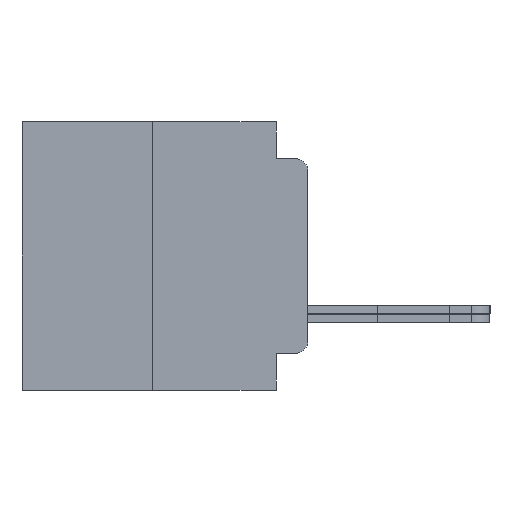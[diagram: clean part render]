
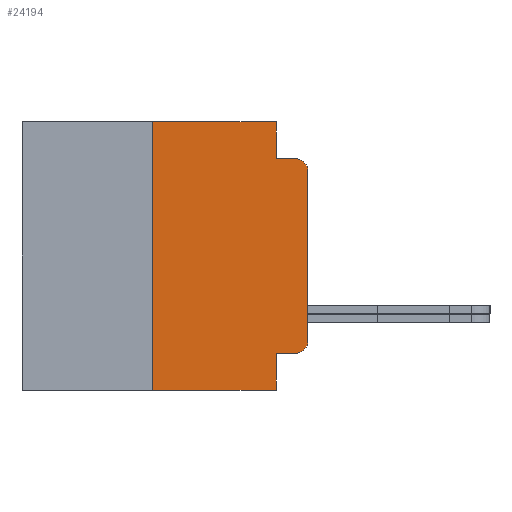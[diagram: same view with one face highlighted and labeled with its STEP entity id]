
A CAD part, left-side view. The second image highlights one B-rep face of the part: STEP entity #24194.
In plain terms, the highlighted planar face has unit normal (-1, 0, 0).
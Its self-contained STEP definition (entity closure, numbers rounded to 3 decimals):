
#92 = CARTESIAN_POINT ( 'NONE',  ( -75.603, 1.295, 0. ) ) ;
#832 = CARTESIAN_POINT ( 'NONE',  ( -75.603, 0., 3.467 ) ) ;
#1432 = DIRECTION ( 'NONE',  ( 1., 0., 0. ) ) ;
#1450 = ORIENTED_EDGE ( 'NONE', *, *, #24512, .F. ) ;
#1784 = VERTEX_POINT ( 'NONE', #21389 ) ;
#1947 = CARTESIAN_POINT ( 'NONE',  ( -75.603, 1.295, -3.975 ) ) ;
#1949 = DIRECTION ( 'NONE',  ( 0., -1., 0. ) ) ;
#2261 = DIRECTION ( 'NONE',  ( 0., 0., -1. ) ) ;
#2635 = VECTOR ( 'NONE', #3875, 1000. ) ;
#3875 = DIRECTION ( 'NONE',  ( 0., 0., -1. ) ) ;
#4479 = CARTESIAN_POINT ( 'NONE',  ( -75.603, 1.295, -3.975 ) ) ;
#4803 = ORIENTED_EDGE ( 'NONE', *, *, #28162, .T. ) ;
#4828 = CARTESIAN_POINT ( 'NONE',  ( -75.603, 6.35, 5.486 ) ) ;
#5490 = DIRECTION ( 'NONE',  ( 0., 0., -1. ) ) ;
#5609 = LINE ( 'NONE', #21966, #27846 ) ;
#6178 = CIRCLE ( 'NONE', #6766, 0.508 ) ;
#6766 = AXIS2_PLACEMENT_3D ( 'NONE', #21391, #14702, #5490 ) ;
#6813 = VERTEX_POINT ( 'NONE', #12914 ) ;
#6880 = VERTEX_POINT ( 'NONE', #13397 ) ;
#7063 = DIRECTION ( 'NONE',  ( 0., -1., 0. ) ) ;
#7454 = ORIENTED_EDGE ( 'NONE', *, *, #24112, .T. ) ;
#7883 = EDGE_CURVE ( 'NONE', #17727, #1784, #21104, .T. ) ;
#8304 = VECTOR ( 'NONE', #10599, 1000. ) ;
#9249 = LINE ( 'NONE', #92, #2635 ) ;
#9313 = VERTEX_POINT ( 'NONE', #4828 ) ;
#9886 = CARTESIAN_POINT ( 'NONE',  ( -75.603, 11.684, -5.486 ) ) ;
#9949 = DIRECTION ( 'NONE',  ( 0., 0., 1. ) ) ;
#10599 = DIRECTION ( 'NONE',  ( 0., 0., 1. ) ) ;
#10908 = LINE ( 'NONE', #23453, #14064 ) ;
#11350 = LINE ( 'NONE', #22685, #26658 ) ;
#11953 = EDGE_LOOP ( 'NONE', ( #20712, #26732, #4803, #14902, #1450, #14119, #21565, #13864, #7454, #24438 ) ) ;
#11989 = VERTEX_POINT ( 'NONE', #12114 ) ;
#12114 = CARTESIAN_POINT ( 'NONE',  ( -75.603, 6.35, -5.486 ) ) ;
#12914 = CARTESIAN_POINT ( 'NONE',  ( -75.603, 0., -3.467 ) ) ;
#13334 = DIRECTION ( 'NONE',  ( -1., 0., 0. ) ) ;
#13397 = CARTESIAN_POINT ( 'NONE',  ( -75.603, 1.295, 5.486 ) ) ;
#13466 = LINE ( 'NONE', #9886, #23875 ) ;
#13689 = CARTESIAN_POINT ( 'NONE',  ( -75.603, 0.508, 3.975 ) ) ;
#13864 = ORIENTED_EDGE ( 'NONE', *, *, #23037, .F. ) ;
#14064 = VECTOR ( 'NONE', #9949, 1000. ) ;
#14099 = EDGE_CURVE ( 'NONE', #9313, #6880, #5609, .T. ) ;
#14119 = ORIENTED_EDGE ( 'NONE', *, *, #16591, .F. ) ;
#14399 = LINE ( 'NONE', #4479, #17189 ) ;
#14702 = DIRECTION ( 'NONE',  ( -1., 0., 0. ) ) ;
#14902 = ORIENTED_EDGE ( 'NONE', *, *, #15928, .T. ) ;
#15517 = VERTEX_POINT ( 'NONE', #832 ) ;
#15559 = DIRECTION ( 'NONE',  ( 0., 0., -1. ) ) ;
#15928 = EDGE_CURVE ( 'NONE', #15517, #16671, #20754, .T. ) ;
#16393 = VERTEX_POINT ( 'NONE', #21714 ) ;
#16591 = EDGE_CURVE ( 'NONE', #6880, #21281, #9249, .T. ) ;
#16671 = VERTEX_POINT ( 'NONE', #13689 ) ;
#16838 = CARTESIAN_POINT ( 'NONE',  ( -75.603, 6.35, -5.486 ) ) ;
#17044 = CARTESIAN_POINT ( 'NONE',  ( -75.603, 1.295, 0. ) ) ;
#17189 = VECTOR ( 'NONE', #1949, 1000. ) ;
#17596 = DIRECTION ( 'NONE',  ( 0., -1., 0. ) ) ;
#17727 = VERTEX_POINT ( 'NONE', #1947 ) ;
#18226 = AXIS2_PLACEMENT_3D ( 'NONE', #26611, #13334, #15559 ) ;
#19005 = PLANE ( 'NONE',  #27965 ) ;
#19101 = DIRECTION ( 'NONE',  ( 0., 0., -1. ) ) ;
#20368 = EDGE_CURVE ( 'NONE', #17727, #16393, #14399, .T. ) ;
#20383 = FACE_OUTER_BOUND ( 'NONE', #11953, .T. ) ;
#20654 = CARTESIAN_POINT ( 'NONE',  ( -75.603, 1.295, 3.975 ) ) ;
#20712 = ORIENTED_EDGE ( 'NONE', *, *, #20368, .T. ) ;
#20754 = CIRCLE ( 'NONE', #18226, 0.508 ) ;
#21104 = LINE ( 'NONE', #17044, #24593 ) ;
#21281 = VERTEX_POINT ( 'NONE', #20654 ) ;
#21389 = CARTESIAN_POINT ( 'NONE',  ( -75.603, 1.295, -5.486 ) ) ;
#21391 = CARTESIAN_POINT ( 'NONE',  ( -75.603, 0.508, -3.467 ) ) ;
#21565 = ORIENTED_EDGE ( 'NONE', *, *, #14099, .F. ) ;
#21714 = CARTESIAN_POINT ( 'NONE',  ( -75.603, 0.508, -3.975 ) ) ;
#21966 = CARTESIAN_POINT ( 'NONE',  ( -75.603, 11.684, 5.486 ) ) ;
#22685 = CARTESIAN_POINT ( 'NONE',  ( -75.603, 1.295, 3.975 ) ) ;
#23037 = EDGE_CURVE ( 'NONE', #11989, #9313, #25327, .T. ) ;
#23453 = CARTESIAN_POINT ( 'NONE',  ( -75.603, 0., 5.486 ) ) ;
#23875 = VECTOR ( 'NONE', #27275, 1000. ) ;
#24112 = EDGE_CURVE ( 'NONE', #11989, #1784, #13466, .T. ) ;
#24194 = ADVANCED_FACE ( 'NONE', ( #20383 ), #19005, .F. ) ;
#24438 = ORIENTED_EDGE ( 'NONE', *, *, #7883, .F. ) ;
#24512 = EDGE_CURVE ( 'NONE', #21281, #16671, #11350, .T. ) ;
#24593 = VECTOR ( 'NONE', #2261, 1000. ) ;
#25327 = LINE ( 'NONE', #16838, #8304 ) ;
#26393 = EDGE_CURVE ( 'NONE', #16393, #6813, #6178, .T. ) ;
#26611 = CARTESIAN_POINT ( 'NONE',  ( -75.603, 0.508, 3.467 ) ) ;
#26658 = VECTOR ( 'NONE', #7063, 1000. ) ;
#26732 = ORIENTED_EDGE ( 'NONE', *, *, #26393, .T. ) ;
#27275 = DIRECTION ( 'NONE',  ( 0., -1., 0. ) ) ;
#27764 = CARTESIAN_POINT ( 'NONE',  ( -75.603, 11.684, 5.486 ) ) ;
#27846 = VECTOR ( 'NONE', #17596, 1000. ) ;
#27965 = AXIS2_PLACEMENT_3D ( 'NONE', #27764, #1432, #19101 ) ;
#28162 = EDGE_CURVE ( 'NONE', #6813, #15517, #10908, .T. ) ;
